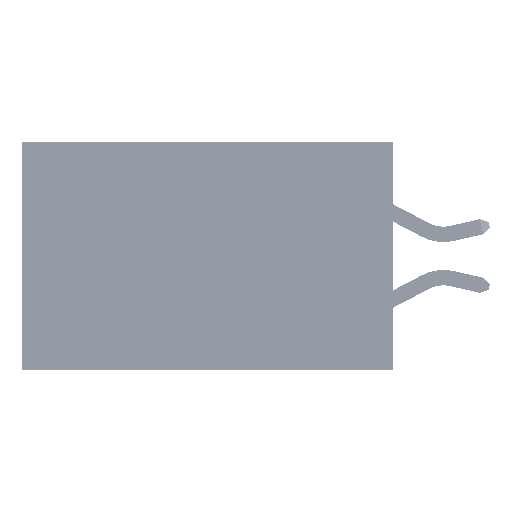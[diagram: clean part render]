
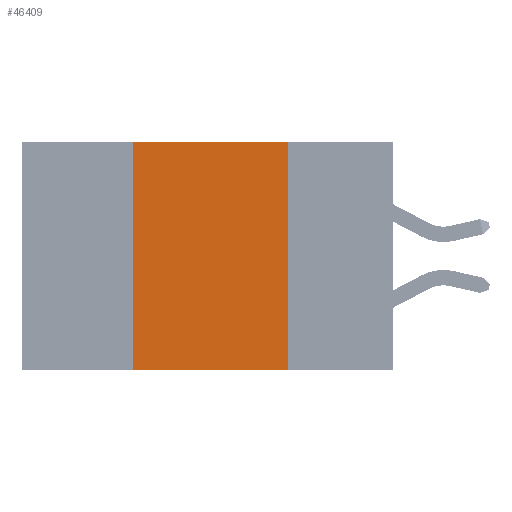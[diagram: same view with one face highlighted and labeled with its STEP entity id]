
A CAD part, left-side view. The second image highlights one B-rep face of the part: STEP entity #46409.
In plain terms, the highlighted planar face has unit normal (-1, 0, 0).
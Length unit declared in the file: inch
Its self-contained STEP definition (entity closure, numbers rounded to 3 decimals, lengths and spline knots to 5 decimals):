
#337 = VERTEX_POINT ( 'NONE', #36915 ) ;
#2072 = CARTESIAN_POINT ( 'NONE',  ( 0., 0.6, 0. ) ) ;
#4923 = ORIENTED_EDGE ( 'NONE', *, *, #45364, .F. ) ;
#5457 = PLANE ( 'NONE',  #47987 ) ;
#6577 = EDGE_CURVE ( 'NONE', #11598, #25017, #49765, .T. ) ;
#6840 = VECTOR ( 'NONE', #32026, 39.37008 ) ;
#7243 = LINE ( 'NONE', #31916, #7262 ) ;
#7262 = VECTOR ( 'NONE', #24111, 39.37008 ) ;
#10868 = VECTOR ( 'NONE', #45363, 39.37008 ) ;
#11598 = VERTEX_POINT ( 'NONE', #30656 ) ;
#11874 = LINE ( 'NONE', #47718, #12064 ) ;
#12064 = VECTOR ( 'NONE', #15251, 39.37008 ) ;
#12538 = LINE ( 'NONE', #39303, #6840 ) ;
#13677 = CARTESIAN_POINT ( 'NONE',  ( 0., 0.17, 0. ) ) ;
#15251 = DIRECTION ( 'NONE',  ( 0., -1., 0. ) ) ;
#17382 = FACE_OUTER_BOUND ( 'NONE', #33958, .T. ) ;
#21550 = DIRECTION ( 'NONE',  ( 1., 0., 0. ) ) ;
#21905 = ORIENTED_EDGE ( 'NONE', *, *, #40512, .T. ) ;
#22324 = DIRECTION ( 'NONE',  ( 0., 0., -1. ) ) ;
#24111 = DIRECTION ( 'NONE',  ( 0., 0., 1. ) ) ;
#25017 = VERTEX_POINT ( 'NONE', #36286 ) ;
#30656 = CARTESIAN_POINT ( 'NONE',  ( 0., 0.17, 0. ) ) ;
#31916 = CARTESIAN_POINT ( 'NONE',  ( 0., 0.42, 0. ) ) ;
#32026 = DIRECTION ( 'NONE',  ( 0., -1., 0. ) ) ;
#33134 = ORIENTED_EDGE ( 'NONE', *, *, #6577, .F. ) ;
#33958 = EDGE_LOOP ( 'NONE', ( #33134, #37638, #4923, #21905 ) ) ;
#35959 = EDGE_CURVE ( 'NONE', #39702, #11598, #12538, .T. ) ;
#36286 = CARTESIAN_POINT ( 'NONE',  ( 0., 0.17, -0.37 ) ) ;
#36915 = CARTESIAN_POINT ( 'NONE',  ( 0., 0.42, -0.37 ) ) ;
#37638 = ORIENTED_EDGE ( 'NONE', *, *, #35959, .F. ) ;
#39303 = CARTESIAN_POINT ( 'NONE',  ( 0., 0.6, 0. ) ) ;
#39702 = VERTEX_POINT ( 'NONE', #47073 ) ;
#40512 = EDGE_CURVE ( 'NONE', #337, #25017, #11874, .T. ) ;
#45363 = DIRECTION ( 'NONE',  ( 0., 0., -1. ) ) ;
#45364 = EDGE_CURVE ( 'NONE', #337, #39702, #7243, .T. ) ;
#46409 = ADVANCED_FACE ( 'NONE', ( #17382 ), #5457, .F. ) ;
#47073 = CARTESIAN_POINT ( 'NONE',  ( 0., 0.42, 0. ) ) ;
#47718 = CARTESIAN_POINT ( 'NONE',  ( 0., 0.6, -0.37 ) ) ;
#47987 = AXIS2_PLACEMENT_3D ( 'NONE', #2072, #21550, #22324 ) ;
#49765 = LINE ( 'NONE', #13677, #10868 ) ;
